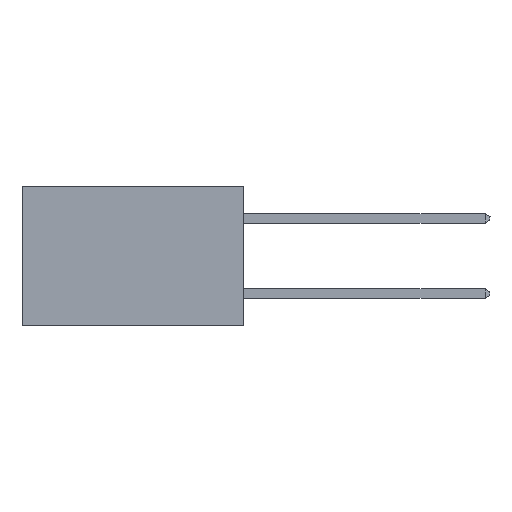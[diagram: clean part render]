
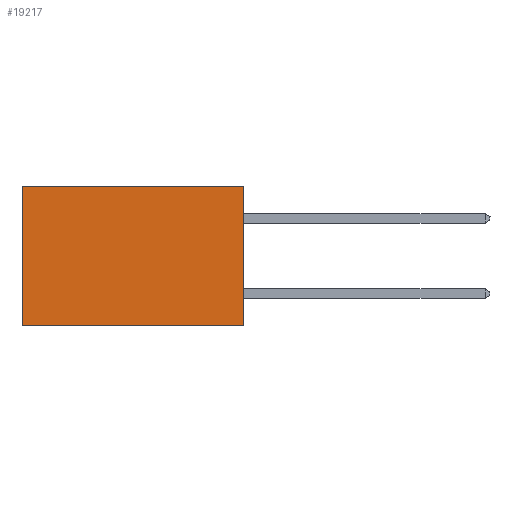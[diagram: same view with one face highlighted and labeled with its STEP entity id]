
A CAD part, left-side view. The second image highlights one B-rep face of the part: STEP entity #19217.
In plain terms, the highlighted planar face has unit normal (-1, 0, 0).
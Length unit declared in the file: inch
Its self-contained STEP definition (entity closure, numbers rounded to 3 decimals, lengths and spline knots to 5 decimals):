
#77 = DIRECTION ( 'NONE',  ( 0., 0., -1. ) ) ;
#235 = EDGE_CURVE ( 'NONE', #5372, #14220, #10279, .T. ) ;
#1107 = VECTOR ( 'NONE', #4394, 39.37008 ) ;
#2721 = CARTESIAN_POINT ( 'NONE',  ( 0.277, 0.59, -0.37 ) ) ;
#3636 = CARTESIAN_POINT ( 'NONE',  ( 0.277, 0.59, -0.37 ) ) ;
#3845 = ORIENTED_EDGE ( 'NONE', *, *, #235, .T. ) ;
#4394 = DIRECTION ( 'NONE',  ( 0., 1., 0. ) ) ;
#4774 = ORIENTED_EDGE ( 'NONE', *, *, #9689, .F. ) ;
#5372 = VERTEX_POINT ( 'NONE', #5407 ) ;
#5407 = CARTESIAN_POINT ( 'NONE',  ( 0.277, 0.59, 0. ) ) ;
#5584 = CARTESIAN_POINT ( 'NONE',  ( 0.277, 0., -0.37 ) ) ;
#6008 = LINE ( 'NONE', #5584, #26887 ) ;
#7477 = VERTEX_POINT ( 'NONE', #16860 ) ;
#9358 = VERTEX_POINT ( 'NONE', #20079 ) ;
#9389 = EDGE_CURVE ( 'NONE', #9358, #5372, #20869, .T. ) ;
#9689 = EDGE_CURVE ( 'NONE', #7477, #14220, #23478, .T. ) ;
#9810 = CARTESIAN_POINT ( 'NONE',  ( 0.277, 0., 0. ) ) ;
#10279 = LINE ( 'NONE', #3636, #20035 ) ;
#10720 = PLANE ( 'NONE',  #24698 ) ;
#11887 = DIRECTION ( 'NONE',  ( 0., 1., 0. ) ) ;
#11940 = EDGE_CURVE ( 'NONE', #9358, #7477, #6008, .T. ) ;
#12730 = CARTESIAN_POINT ( 'NONE',  ( 0.277, 0., -0.37 ) ) ;
#12823 = DIRECTION ( 'NONE',  ( 1., 0., 0. ) ) ;
#14220 = VERTEX_POINT ( 'NONE', #2721 ) ;
#16032 = DIRECTION ( 'NONE',  ( 0., 0., -1. ) ) ;
#16860 = CARTESIAN_POINT ( 'NONE',  ( 0.277, 0., -0.37 ) ) ;
#19217 = ADVANCED_FACE ( 'NONE', ( #25787 ), #10720, .F. ) ;
#19894 = EDGE_LOOP ( 'NONE', ( #3845, #4774, #24702, #26708 ) ) ;
#20035 = VECTOR ( 'NONE', #20453, 39.37008 ) ;
#20079 = CARTESIAN_POINT ( 'NONE',  ( 0.277, 0., 0. ) ) ;
#20453 = DIRECTION ( 'NONE',  ( 0., 0., -1. ) ) ;
#20869 = LINE ( 'NONE', #9810, #25104 ) ;
#23143 = CARTESIAN_POINT ( 'NONE',  ( 0.277, 0., -0.37 ) ) ;
#23478 = LINE ( 'NONE', #23143, #1107 ) ;
#24698 = AXIS2_PLACEMENT_3D ( 'NONE', #12730, #12823, #77 ) ;
#24702 = ORIENTED_EDGE ( 'NONE', *, *, #11940, .F. ) ;
#25104 = VECTOR ( 'NONE', #11887, 39.37008 ) ;
#25787 = FACE_OUTER_BOUND ( 'NONE', #19894, .T. ) ;
#26708 = ORIENTED_EDGE ( 'NONE', *, *, #9389, .T. ) ;
#26887 = VECTOR ( 'NONE', #16032, 39.37008 ) ;
